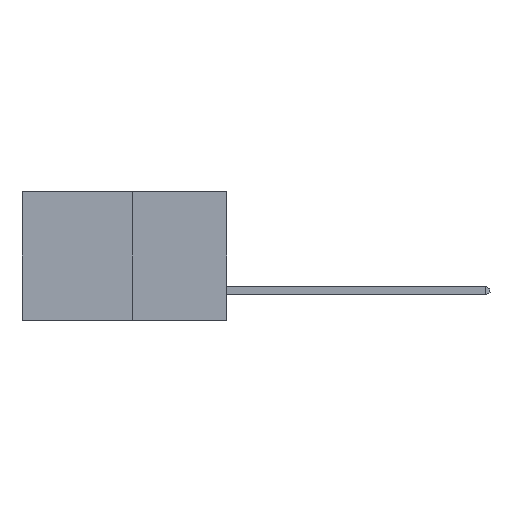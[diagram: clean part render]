
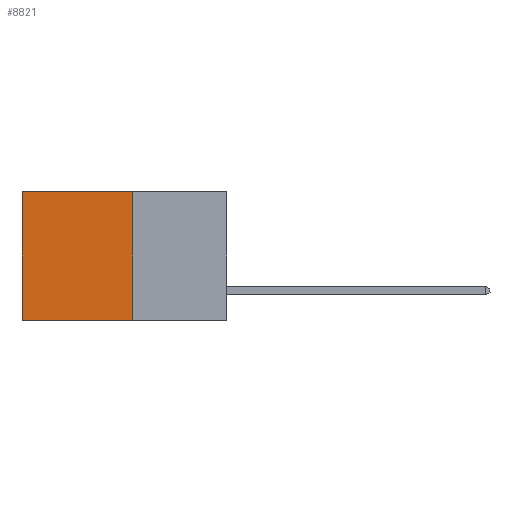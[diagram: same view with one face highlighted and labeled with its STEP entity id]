
A CAD part, left-side view. The second image highlights one B-rep face of the part: STEP entity #8821.
In plain terms, the highlighted planar face has unit normal (-1, 0, 0).
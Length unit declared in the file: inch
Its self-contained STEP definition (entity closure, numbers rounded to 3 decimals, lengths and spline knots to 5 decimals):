
#135 = AXIS2_PLACEMENT_3D ( 'NONE', #6499, #2297, #7190 ) ;
#286 = DIRECTION ( 'NONE',  ( 0., 0., -1. ) ) ;
#1105 = VERTEX_POINT ( 'NONE', #4662 ) ;
#1407 = VECTOR ( 'NONE', #5715, 39.37008 ) ;
#1574 = VERTEX_POINT ( 'NONE', #3176 ) ;
#1801 = EDGE_CURVE ( 'NONE', #1105, #4445, #5458, .T. ) ;
#1848 = LINE ( 'NONE', #5472, #1407 ) ;
#2051 = ORIENTED_EDGE ( 'NONE', *, *, #4085, .F. ) ;
#2297 = DIRECTION ( 'NONE',  ( 1., 0., 0. ) ) ;
#2445 = DIRECTION ( 'NONE',  ( 0., 0., -1. ) ) ;
#2965 = EDGE_LOOP ( 'NONE', ( #7326, #2051, #5373, #3048 ) ) ;
#3048 = ORIENTED_EDGE ( 'NONE', *, *, #4021, .T. ) ;
#3176 = CARTESIAN_POINT ( 'NONE',  ( 0.277, 0.27, -0.37 ) ) ;
#3715 = PLANE ( 'NONE',  #135 ) ;
#3765 = VECTOR ( 'NONE', #4754, 39.37008 ) ;
#3802 = CARTESIAN_POINT ( 'NONE',  ( 0.277, 0.27, -0.37 ) ) ;
#4021 = EDGE_CURVE ( 'NONE', #7587, #1105, #7430, .T. ) ;
#4085 = EDGE_CURVE ( 'NONE', #1574, #4445, #1848, .T. ) ;
#4445 = VERTEX_POINT ( 'NONE', #7626 ) ;
#4662 = CARTESIAN_POINT ( 'NONE',  ( 0.277, 0.59, 0. ) ) ;
#4754 = DIRECTION ( 'NONE',  ( 0., 1., 0. ) ) ;
#4809 = FACE_OUTER_BOUND ( 'NONE', #2965, .T. ) ;
#5055 = EDGE_CURVE ( 'NONE', #7587, #1574, #7523, .T. ) ;
#5373 = ORIENTED_EDGE ( 'NONE', *, *, #5055, .F. ) ;
#5458 = LINE ( 'NONE', #8625, #6841 ) ;
#5472 = CARTESIAN_POINT ( 'NONE',  ( 0.277, 0.27, -0.37 ) ) ;
#5715 = DIRECTION ( 'NONE',  ( 0., 1., 0. ) ) ;
#6191 = CARTESIAN_POINT ( 'NONE',  ( 0.277, 0.27, 0. ) ) ;
#6379 = CARTESIAN_POINT ( 'NONE',  ( 0.277, 0.27, 0. ) ) ;
#6499 = CARTESIAN_POINT ( 'NONE',  ( 0.277, 0.27, -0.37 ) ) ;
#6841 = VECTOR ( 'NONE', #2445, 39.37008 ) ;
#7190 = DIRECTION ( 'NONE',  ( 0., 0., -1. ) ) ;
#7309 = VECTOR ( 'NONE', #286, 39.37008 ) ;
#7326 = ORIENTED_EDGE ( 'NONE', *, *, #1801, .T. ) ;
#7430 = LINE ( 'NONE', #6191, #3765 ) ;
#7523 = LINE ( 'NONE', #3802, #7309 ) ;
#7587 = VERTEX_POINT ( 'NONE', #6379 ) ;
#7626 = CARTESIAN_POINT ( 'NONE',  ( 0.277, 0.59, -0.37 ) ) ;
#8625 = CARTESIAN_POINT ( 'NONE',  ( 0.277, 0.59, -0.37 ) ) ;
#8821 = ADVANCED_FACE ( 'NONE', ( #4809 ), #3715, .F. ) ;
